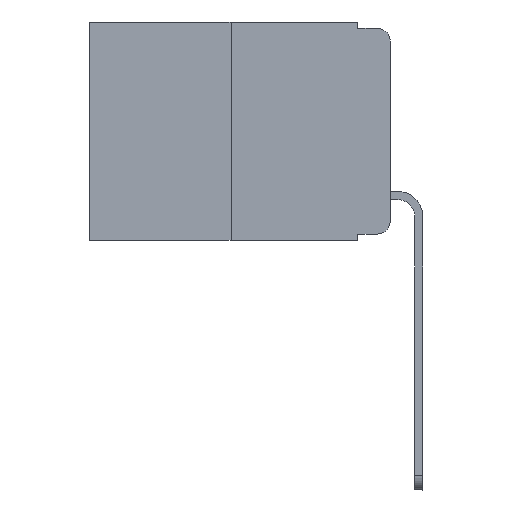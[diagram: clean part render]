
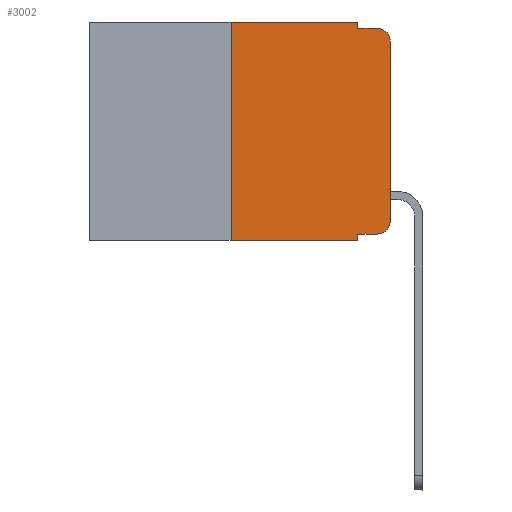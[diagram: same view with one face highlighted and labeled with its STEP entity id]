
A CAD part, left-side view. The second image highlights one B-rep face of the part: STEP entity #3002.
In plain terms, the highlighted planar face has unit normal (-1, 0, 0).
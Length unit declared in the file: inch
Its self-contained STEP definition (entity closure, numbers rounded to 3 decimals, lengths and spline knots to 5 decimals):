
#11 = ORIENTED_EDGE ( 'NONE', *, *, #10626, .T. ) ;
#215 = EDGE_CURVE ( 'NONE', #7461, #16989, #18108, .T. ) ;
#444 = DIRECTION ( 'NONE',  ( 0., 0., -1. ) ) ;
#559 = VERTEX_POINT ( 'NONE', #5431 ) ;
#571 = VERTEX_POINT ( 'NONE', #10007 ) ;
#1041 = CARTESIAN_POINT ( 'NONE',  ( 0., 0., 0. ) ) ;
#1755 = DIRECTION ( 'NONE',  ( 0., -1., 0. ) ) ;
#1762 = DIRECTION ( 'NONE',  ( 0., 0., -1. ) ) ;
#1939 = EDGE_LOOP ( 'NONE', ( #11, #16731, #19012, #8852, #11830, #8807, #17329, #4332, #4144, #12031 ) ) ;
#2209 = CARTESIAN_POINT ( 'NONE',  ( 0., 0.02, -0.01 ) ) ;
#2705 = AXIS2_PLACEMENT_3D ( 'NONE', #15756, #14352, #444 ) ;
#3002 = ADVANCED_FACE ( 'NONE', ( #11519 ), #3849, .F. ) ;
#3441 = CARTESIAN_POINT ( 'NONE',  ( 0., 0.02, -0.333 ) ) ;
#3787 = VERTEX_POINT ( 'NONE', #7409 ) ;
#3849 = PLANE ( 'NONE',  #13366 ) ;
#3899 = DIRECTION ( 'NONE',  ( 0., 0., 1. ) ) ;
#3945 = VECTOR ( 'NONE', #5649, 39.37008 ) ;
#4015 = DIRECTION ( 'NONE',  ( 0., 0., 1. ) ) ;
#4144 = ORIENTED_EDGE ( 'NONE', *, *, #13005, .T. ) ;
#4160 = EDGE_CURVE ( 'NONE', #19535, #559, #18247, .T. ) ;
#4332 = ORIENTED_EDGE ( 'NONE', *, *, #4160, .F. ) ;
#4489 = CARTESIAN_POINT ( 'NONE',  ( 0., 0.051, 0. ) ) ;
#4664 = DIRECTION ( 'NONE',  ( 0., 0., -1. ) ) ;
#4909 = LINE ( 'NONE', #6495, #7829 ) ;
#4980 = CARTESIAN_POINT ( 'NONE',  ( 0., 0.473, 0. ) ) ;
#5372 = DIRECTION ( 'NONE',  ( 0., -1., 0. ) ) ;
#5380 = VECTOR ( 'NONE', #19645, 39.37008 ) ;
#5431 = CARTESIAN_POINT ( 'NONE',  ( 0., 0.051, -0.343 ) ) ;
#5435 = VERTEX_POINT ( 'NONE', #6104 ) ;
#5510 = VECTOR ( 'NONE', #4015, 39.37008 ) ;
#5649 = DIRECTION ( 'NONE',  ( 0., -1., 0. ) ) ;
#6104 = CARTESIAN_POINT ( 'NONE',  ( 0., 0., -0.03 ) ) ;
#6193 = AXIS2_PLACEMENT_3D ( 'NONE', #9444, #15416, #4664 ) ;
#6432 = CARTESIAN_POINT ( 'NONE',  ( 0., 0.051, -0.333 ) ) ;
#6490 = EDGE_CURVE ( 'NONE', #3787, #7461, #15403, .T. ) ;
#6495 = CARTESIAN_POINT ( 'NONE',  ( 0., 0.473, 0. ) ) ;
#6958 = LINE ( 'NONE', #9957, #8968 ) ;
#7165 = LINE ( 'NONE', #13255, #8835 ) ;
#7409 = CARTESIAN_POINT ( 'NONE',  ( 0., 0.051, 0. ) ) ;
#7461 = VERTEX_POINT ( 'NONE', #10411 ) ;
#7829 = VECTOR ( 'NONE', #8071, 39.37008 ) ;
#8071 = DIRECTION ( 'NONE',  ( 0., -1., 0. ) ) ;
#8807 = ORIENTED_EDGE ( 'NONE', *, *, #18435, .F. ) ;
#8835 = VECTOR ( 'NONE', #3899, 39.37008 ) ;
#8852 = ORIENTED_EDGE ( 'NONE', *, *, #6490, .F. ) ;
#8968 = VECTOR ( 'NONE', #5372, 39.37008 ) ;
#9429 = CARTESIAN_POINT ( 'NONE',  ( 0., 0.051, 0. ) ) ;
#9444 = CARTESIAN_POINT ( 'NONE',  ( 0., 0.02, -0.313 ) ) ;
#9557 = DIRECTION ( 'NONE',  ( 1., 0., 0. ) ) ;
#9821 = EDGE_CURVE ( 'NONE', #13358, #559, #6958, .T. ) ;
#9957 = CARTESIAN_POINT ( 'NONE',  ( 0., 0.473, -0.343 ) ) ;
#10007 = CARTESIAN_POINT ( 'NONE',  ( 0., 0., -0.313 ) ) ;
#10411 = CARTESIAN_POINT ( 'NONE',  ( 0., 0.051, -0.01 ) ) ;
#10626 = EDGE_CURVE ( 'NONE', #571, #5435, #16165, .T. ) ;
#11519 = FACE_OUTER_BOUND ( 'NONE', #1939, .T. ) ;
#11830 = ORIENTED_EDGE ( 'NONE', *, *, #15587, .F. ) ;
#12031 = ORIENTED_EDGE ( 'NONE', *, *, #12598, .T. ) ;
#12214 = LINE ( 'NONE', #6432, #14471 ) ;
#12257 = CIRCLE ( 'NONE', #6193, 0.02 ) ;
#12392 = EDGE_CURVE ( 'NONE', #5435, #16989, #16053, .T. ) ;
#12598 = EDGE_CURVE ( 'NONE', #13082, #571, #12257, .T. ) ;
#13005 = EDGE_CURVE ( 'NONE', #19535, #13082, #12214, .T. ) ;
#13082 = VERTEX_POINT ( 'NONE', #3441 ) ;
#13255 = CARTESIAN_POINT ( 'NONE',  ( 0., 0.25, 0. ) ) ;
#13358 = VERTEX_POINT ( 'NONE', #17881 ) ;
#13366 = AXIS2_PLACEMENT_3D ( 'NONE', #4980, #9557, #18995 ) ;
#13456 = VERTEX_POINT ( 'NONE', #13871 ) ;
#13871 = CARTESIAN_POINT ( 'NONE',  ( 0., 0.25, 0. ) ) ;
#14352 = DIRECTION ( 'NONE',  ( -1., 0., 0. ) ) ;
#14469 = CARTESIAN_POINT ( 'NONE',  ( 0., 0.051, -0.333 ) ) ;
#14471 = VECTOR ( 'NONE', #1755, 39.37008 ) ;
#15403 = LINE ( 'NONE', #9429, #16864 ) ;
#15416 = DIRECTION ( 'NONE',  ( -1., 0., 0. ) ) ;
#15587 = EDGE_CURVE ( 'NONE', #13456, #3787, #4909, .T. ) ;
#15756 = CARTESIAN_POINT ( 'NONE',  ( 0., 0.02, -0.03 ) ) ;
#16053 = CIRCLE ( 'NONE', #2705, 0.02 ) ;
#16165 = LINE ( 'NONE', #1041, #5510 ) ;
#16731 = ORIENTED_EDGE ( 'NONE', *, *, #12392, .T. ) ;
#16864 = VECTOR ( 'NONE', #1762, 39.37008 ) ;
#16989 = VERTEX_POINT ( 'NONE', #2209 ) ;
#17329 = ORIENTED_EDGE ( 'NONE', *, *, #9821, .T. ) ;
#17881 = CARTESIAN_POINT ( 'NONE',  ( 0., 0.25, -0.343 ) ) ;
#17916 = CARTESIAN_POINT ( 'NONE',  ( 0., 0.051, -0.01 ) ) ;
#18108 = LINE ( 'NONE', #17916, #3945 ) ;
#18247 = LINE ( 'NONE', #4489, #5380 ) ;
#18435 = EDGE_CURVE ( 'NONE', #13358, #13456, #7165, .T. ) ;
#18995 = DIRECTION ( 'NONE',  ( 0., 0., -1. ) ) ;
#19012 = ORIENTED_EDGE ( 'NONE', *, *, #215, .F. ) ;
#19535 = VERTEX_POINT ( 'NONE', #14469 ) ;
#19645 = DIRECTION ( 'NONE',  ( 0., 0., -1. ) ) ;
